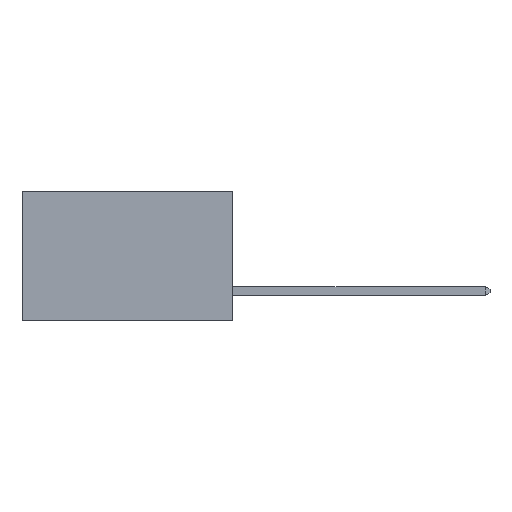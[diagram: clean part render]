
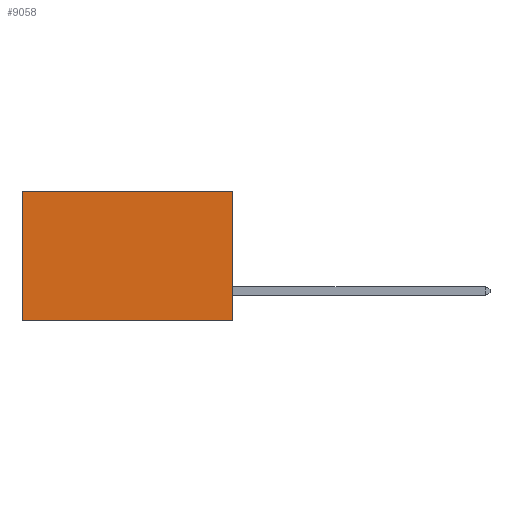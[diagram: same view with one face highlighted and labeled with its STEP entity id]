
A CAD part, left-side view. The second image highlights one B-rep face of the part: STEP entity #9058.
In plain terms, the highlighted planar face has unit normal (-1, 0, 0).
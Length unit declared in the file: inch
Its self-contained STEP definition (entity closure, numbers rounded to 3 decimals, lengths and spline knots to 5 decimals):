
#117 = ORIENTED_EDGE ( 'NONE', *, *, #2205, .T. ) ;
#132 = LINE ( 'NONE', #10942, #9273 ) ;
#217 = CARTESIAN_POINT ( 'NONE',  ( 0.2875, 0., 0. ) ) ;
#1267 = EDGE_CURVE ( 'NONE', #15074, #4596, #12074, .T. ) ;
#1459 = EDGE_CURVE ( 'NONE', #10214, #15074, #132, .T. ) ;
#2205 = EDGE_CURVE ( 'NONE', #13219, #4596, #12566, .T. ) ;
#2456 = LINE ( 'NONE', #217, #6925 ) ;
#3342 = CARTESIAN_POINT ( 'NONE',  ( 0.2875, 0., -0.37 ) ) ;
#3453 = VECTOR ( 'NONE', #7656, 39.37008 ) ;
#3649 = ORIENTED_EDGE ( 'NONE', *, *, #1267, .F. ) ;
#4248 = PLANE ( 'NONE',  #9740 ) ;
#4596 = VERTEX_POINT ( 'NONE', #13983 ) ;
#5090 = DIRECTION ( 'NONE',  ( 0., 0., -1. ) ) ;
#5497 = DIRECTION ( 'NONE',  ( 1., 0., 0. ) ) ;
#5727 = ORIENTED_EDGE ( 'NONE', *, *, #13721, .T. ) ;
#6375 = DIRECTION ( 'NONE',  ( 0., 1., 0. ) ) ;
#6829 = EDGE_LOOP ( 'NONE', ( #117, #3649, #8704, #5727 ) ) ;
#6925 = VECTOR ( 'NONE', #6375, 39.37008 ) ;
#7656 = DIRECTION ( 'NONE',  ( 0., 0., -1. ) ) ;
#7937 = CARTESIAN_POINT ( 'NONE',  ( 0.2875, 0.6, 0. ) ) ;
#8704 = ORIENTED_EDGE ( 'NONE', *, *, #1459, .F. ) ;
#8771 = VECTOR ( 'NONE', #8827, 39.37008 ) ;
#8787 = CARTESIAN_POINT ( 'NONE',  ( 0.2875, 0., 0. ) ) ;
#8827 = DIRECTION ( 'NONE',  ( 0., 1., 0. ) ) ;
#8902 = CARTESIAN_POINT ( 'NONE',  ( 0.2875, 0.6, 0. ) ) ;
#9058 = ADVANCED_FACE ( 'NONE', ( #14280 ), #4248, .F. ) ;
#9273 = VECTOR ( 'NONE', #5090, 39.37008 ) ;
#9740 = AXIS2_PLACEMENT_3D ( 'NONE', #12164, #5497, #13322 ) ;
#10066 = CARTESIAN_POINT ( 'NONE',  ( 0.2875, 0., -0.37 ) ) ;
#10214 = VERTEX_POINT ( 'NONE', #8787 ) ;
#10942 = CARTESIAN_POINT ( 'NONE',  ( 0.2875, 0., 0. ) ) ;
#12074 = LINE ( 'NONE', #10066, #8771 ) ;
#12164 = CARTESIAN_POINT ( 'NONE',  ( 0.2875, 0., 0. ) ) ;
#12566 = LINE ( 'NONE', #7937, #3453 ) ;
#13219 = VERTEX_POINT ( 'NONE', #8902 ) ;
#13322 = DIRECTION ( 'NONE',  ( 0., 0., -1. ) ) ;
#13721 = EDGE_CURVE ( 'NONE', #10214, #13219, #2456, .T. ) ;
#13983 = CARTESIAN_POINT ( 'NONE',  ( 0.2875, 0.6, -0.37 ) ) ;
#14280 = FACE_OUTER_BOUND ( 'NONE', #6829, .T. ) ;
#15074 = VERTEX_POINT ( 'NONE', #3342 ) ;
